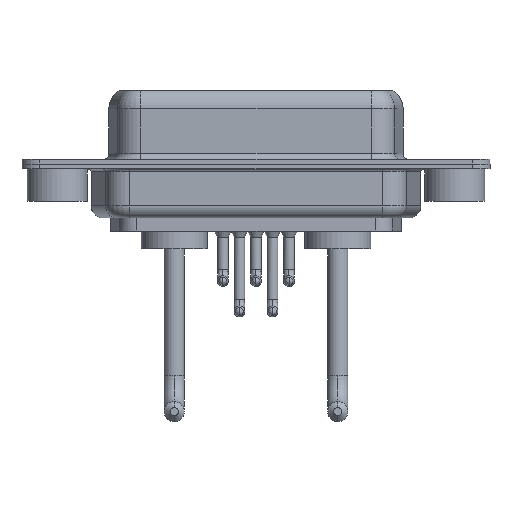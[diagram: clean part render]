
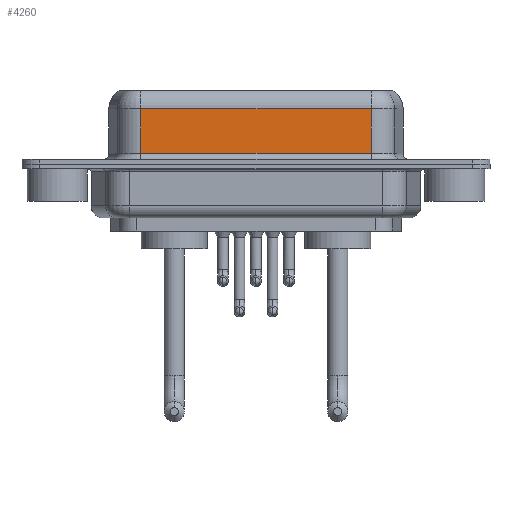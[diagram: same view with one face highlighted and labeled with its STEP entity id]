
A CAD part, front view. The second image highlights one B-rep face of the part: STEP entity #4260.
In plain terms, the highlighted planar face has unit normal (0, -1, 0).
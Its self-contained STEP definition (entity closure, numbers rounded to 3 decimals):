
#150 = DIRECTION ( 'NONE',  ( 1., 0., 0. ) ) ;
#436 = CARTESIAN_POINT ( 'NONE',  ( 7.013, -3.95, 6.4 ) ) ;
#738 = DIRECTION ( 'NONE',  ( 0., 1., 0. ) ) ;
#753 = VERTEX_POINT ( 'NONE', #7610 ) ;
#1378 = DIRECTION ( 'NONE',  ( 0., 0., -1. ) ) ;
#2260 = FACE_OUTER_BOUND ( 'NONE', #12968, .T. ) ;
#2333 = EDGE_CURVE ( 'NONE', #753, #4997, #12947, .T. ) ;
#2755 = CARTESIAN_POINT ( 'NONE',  ( 26.287, -3.95, 0.9 ) ) ;
#3131 = ORIENTED_EDGE ( 'NONE', *, *, #2333, .T. ) ;
#3474 = EDGE_CURVE ( 'NONE', #5223, #753, #4288, .T. ) ;
#4145 = VERTEX_POINT ( 'NONE', #7841 ) ;
#4260 = ADVANCED_FACE ( 'NONE', ( #2260 ), #11406, .F. ) ;
#4288 = LINE ( 'NONE', #436, #7011 ) ;
#4997 = VERTEX_POINT ( 'NONE', #2755 ) ;
#5223 = VERTEX_POINT ( 'NONE', #16271 ) ;
#6690 = CARTESIAN_POINT ( 'NONE',  ( 26.287, -3.95, 6.4 ) ) ;
#6970 = ORIENTED_EDGE ( 'NONE', *, *, #8307, .F. ) ;
#7011 = VECTOR ( 'NONE', #13468, 1000. ) ;
#7610 = CARTESIAN_POINT ( 'NONE',  ( 7.013, -3.95, 0.9 ) ) ;
#7667 = CARTESIAN_POINT ( 'NONE',  ( 26.287, -3.95, 0.9 ) ) ;
#7841 = CARTESIAN_POINT ( 'NONE',  ( 26.287, -3.95, 4.65 ) ) ;
#7904 = VECTOR ( 'NONE', #1378, 1000. ) ;
#8307 = EDGE_CURVE ( 'NONE', #4145, #4997, #10436, .T. ) ;
#8639 = DIRECTION ( 'NONE',  ( -1., 0., 0. ) ) ;
#8806 = CARTESIAN_POINT ( 'NONE',  ( 26.287, -3.95, 4.65 ) ) ;
#9311 = EDGE_CURVE ( 'NONE', #4145, #5223, #12728, .T. ) ;
#10436 = LINE ( 'NONE', #6690, #7904 ) ;
#10499 = VECTOR ( 'NONE', #150, 1000. ) ;
#10977 = AXIS2_PLACEMENT_3D ( 'NONE', #12427, #738, #15401 ) ;
#11406 = PLANE ( 'NONE',  #10977 ) ;
#12427 = CARTESIAN_POINT ( 'NONE',  ( 26.287, -3.95, 6.4 ) ) ;
#12624 = ORIENTED_EDGE ( 'NONE', *, *, #9311, .T. ) ;
#12728 = LINE ( 'NONE', #8806, #14397 ) ;
#12947 = LINE ( 'NONE', #7667, #10499 ) ;
#12968 = EDGE_LOOP ( 'NONE', ( #6970, #12624, #13313, #3131 ) ) ;
#13313 = ORIENTED_EDGE ( 'NONE', *, *, #3474, .T. ) ;
#13468 = DIRECTION ( 'NONE',  ( 0., 0., -1. ) ) ;
#14397 = VECTOR ( 'NONE', #8639, 1000. ) ;
#15401 = DIRECTION ( 'NONE',  ( 0., 0., 1. ) ) ;
#16271 = CARTESIAN_POINT ( 'NONE',  ( 7.013, -3.95, 4.65 ) ) ;
